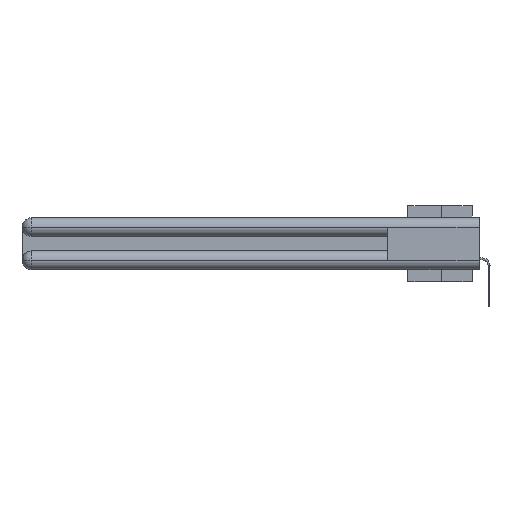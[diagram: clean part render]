
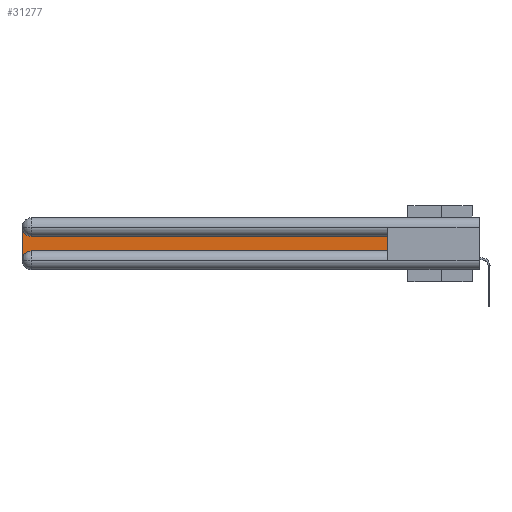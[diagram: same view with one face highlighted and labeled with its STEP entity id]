
A CAD part, left-side view. The second image highlights one B-rep face of the part: STEP entity #31277.
In plain terms, the highlighted planar face has unit normal (-1, 0, 0).
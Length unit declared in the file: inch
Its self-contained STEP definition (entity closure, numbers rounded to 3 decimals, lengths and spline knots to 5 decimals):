
#264 = CARTESIAN_POINT ( 'NONE',  ( 0.075, 2.94, -0.1225 ) ) ;
#643 = ORIENTED_EDGE ( 'NONE', *, *, #31018, .T. ) ;
#1308 = VERTEX_POINT ( 'NONE', #28469 ) ;
#1542 = EDGE_CURVE ( 'NONE', #8676, #4001, #11224, .T. ) ;
#2459 = EDGE_CURVE ( 'NONE', #1308, #3407, #28833, .T. ) ;
#3407 = VERTEX_POINT ( 'NONE', #15223 ) ;
#3902 = CARTESIAN_POINT ( 'NONE',  ( 0.075, 3., -0.1225 ) ) ;
#4001 = VERTEX_POINT ( 'NONE', #17889 ) ;
#4642 = EDGE_CURVE ( 'NONE', #4001, #1308, #19578, .T. ) ;
#5906 = VECTOR ( 'NONE', #22281, 39.37008 ) ;
#6716 = DIRECTION ( 'NONE',  ( 0., 0., -1. ) ) ;
#7337 = CARTESIAN_POINT ( 'NONE',  ( 0.075, 2.94, -0.0625 ) ) ;
#8029 = CARTESIAN_POINT ( 'NONE',  ( 0.075, 0.6, -0.2175 ) ) ;
#8676 = VERTEX_POINT ( 'NONE', #264 ) ;
#8967 = PLANE ( 'NONE',  #24266 ) ;
#9225 = VECTOR ( 'NONE', #12182, 39.37008 ) ;
#9679 = EDGE_LOOP ( 'NONE', ( #11746, #18873, #28955, #11542, #643, #30869 ) ) ;
#11199 = DIRECTION ( 'NONE',  ( 0., 0., -1. ) ) ;
#11224 = CIRCLE ( 'NONE', #13245, 0.06 ) ;
#11542 = ORIENTED_EDGE ( 'NONE', *, *, #2459, .T. ) ;
#11746 = ORIENTED_EDGE ( 'NONE', *, *, #30841, .T. ) ;
#11907 = LINE ( 'NONE', #31305, #12088 ) ;
#12059 = DIRECTION ( 'NONE',  ( 0., 1., 0. ) ) ;
#12088 = VECTOR ( 'NONE', #12059, 39.37008 ) ;
#12182 = DIRECTION ( 'NONE',  ( 0., 0., 1. ) ) ;
#12592 = VECTOR ( 'NONE', #25181, 39.37008 ) ;
#12928 = VERTEX_POINT ( 'NONE', #21097 ) ;
#13245 = AXIS2_PLACEMENT_3D ( 'NONE', #7337, #26557, #25065 ) ;
#13310 = VERTEX_POINT ( 'NONE', #25499 ) ;
#14946 = CARTESIAN_POINT ( 'NONE',  ( 0.075, 3., -0.2175 ) ) ;
#15223 = CARTESIAN_POINT ( 'NONE',  ( 0.075, 2.94, -0.2175 ) ) ;
#17263 = CARTESIAN_POINT ( 'NONE',  ( 0.075, 0.6, -0.2175 ) ) ;
#17390 = EDGE_CURVE ( 'NONE', #12928, #13310, #23951, .T. ) ;
#17889 = CARTESIAN_POINT ( 'NONE',  ( 0.075, 3., -0.0625 ) ) ;
#18671 = DIRECTION ( 'NONE',  ( 1., 0., 0. ) ) ;
#18873 = ORIENTED_EDGE ( 'NONE', *, *, #1542, .T. ) ;
#19199 = AXIS2_PLACEMENT_3D ( 'NONE', #28323, #28798, #6716 ) ;
#19578 = LINE ( 'NONE', #14946, #5906 ) ;
#21097 = CARTESIAN_POINT ( 'NONE',  ( 0.075, 0.6, -0.2175 ) ) ;
#22281 = DIRECTION ( 'NONE',  ( 0., 0., -1. ) ) ;
#23951 = LINE ( 'NONE', #17263, #9225 ) ;
#24266 = AXIS2_PLACEMENT_3D ( 'NONE', #3902, #18671, #11199 ) ;
#25012 = LINE ( 'NONE', #8029, #12592 ) ;
#25065 = DIRECTION ( 'NONE',  ( 0., 0., -1. ) ) ;
#25181 = DIRECTION ( 'NONE',  ( 0., -1., 0. ) ) ;
#25499 = CARTESIAN_POINT ( 'NONE',  ( 0.075, 0.6, -0.1225 ) ) ;
#25652 = FACE_OUTER_BOUND ( 'NONE', #9679, .T. ) ;
#26557 = DIRECTION ( 'NONE',  ( 1., 0., 0. ) ) ;
#28323 = CARTESIAN_POINT ( 'NONE',  ( 0.075, 2.94, -0.2775 ) ) ;
#28469 = CARTESIAN_POINT ( 'NONE',  ( 0.075, 3., -0.2775 ) ) ;
#28798 = DIRECTION ( 'NONE',  ( 1., 0., 0. ) ) ;
#28833 = CIRCLE ( 'NONE', #19199, 0.06 ) ;
#28955 = ORIENTED_EDGE ( 'NONE', *, *, #4642, .T. ) ;
#30841 = EDGE_CURVE ( 'NONE', #13310, #8676, #11907, .T. ) ;
#30869 = ORIENTED_EDGE ( 'NONE', *, *, #17390, .T. ) ;
#31018 = EDGE_CURVE ( 'NONE', #3407, #12928, #25012, .T. ) ;
#31277 = ADVANCED_FACE ( 'NONE', ( #25652 ), #8967, .F. ) ;
#31305 = CARTESIAN_POINT ( 'NONE',  ( 0.075, 0.6, -0.1225 ) ) ;
